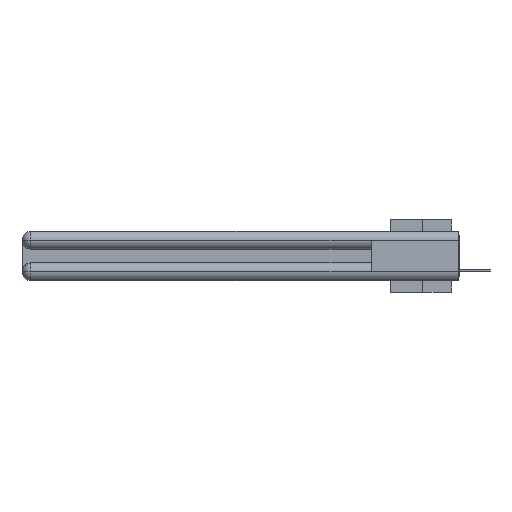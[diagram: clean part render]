
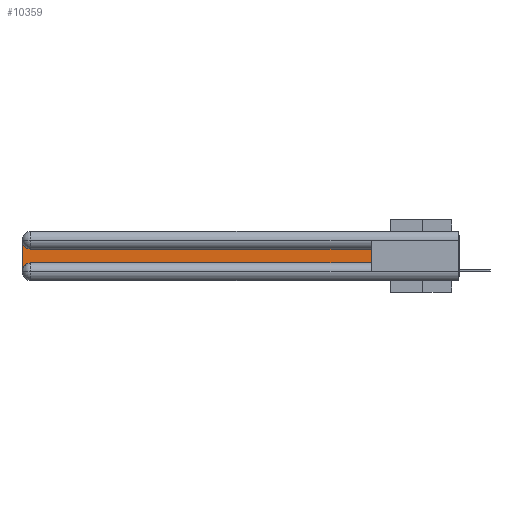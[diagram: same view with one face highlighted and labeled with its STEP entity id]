
A CAD part, left-side view. The second image highlights one B-rep face of the part: STEP entity #10359.
In plain terms, the highlighted planar face has unit normal (-1, 0, 0).
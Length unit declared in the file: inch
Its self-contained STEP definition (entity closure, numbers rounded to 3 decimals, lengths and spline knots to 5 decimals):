
#188 = CARTESIAN_POINT ( 'NONE',  ( 0.075, 3., -0.2175 ) ) ;
#963 = ORIENTED_EDGE ( 'NONE', *, *, #7493, .T. ) ;
#1847 = CARTESIAN_POINT ( 'NONE',  ( 0.075, 2.94, -0.2775 ) ) ;
#2055 = DIRECTION ( 'NONE',  ( 1., 0., 0. ) ) ;
#2234 = LINE ( 'NONE', #188, #9024 ) ;
#4296 = EDGE_CURVE ( 'NONE', #28843, #17159, #2234, .T. ) ;
#6212 = ORIENTED_EDGE ( 'NONE', *, *, #6894, .T. ) ;
#6613 = DIRECTION ( 'NONE',  ( 0., 1., 0. ) ) ;
#6894 = EDGE_CURVE ( 'NONE', #22599, #12963, #25874, .T. ) ;
#7059 = CARTESIAN_POINT ( 'NONE',  ( 0.075, 0.6, -0.2175 ) ) ;
#7493 = EDGE_CURVE ( 'NONE', #19173, #12320, #16929, .T. ) ;
#7584 = LINE ( 'NONE', #29138, #8318 ) ;
#8318 = VECTOR ( 'NONE', #17088, 39.37008 ) ;
#8584 = ORIENTED_EDGE ( 'NONE', *, *, #4296, .T. ) ;
#8745 = DIRECTION ( 'NONE',  ( 0., 0., -1. ) ) ;
#8918 = EDGE_CURVE ( 'NONE', #12320, #28843, #13031, .T. ) ;
#9024 = VECTOR ( 'NONE', #19634, 39.37008 ) ;
#10276 = CARTESIAN_POINT ( 'NONE',  ( 0.075, 0.6, -0.1225 ) ) ;
#10359 = ADVANCED_FACE ( 'NONE', ( #26629 ), #30049, .F. ) ;
#11123 = CARTESIAN_POINT ( 'NONE',  ( 0.075, 3., -0.1225 ) ) ;
#11549 = EDGE_LOOP ( 'NONE', ( #963, #23551, #8584, #31205, #6212, #21942 ) ) ;
#12320 = VERTEX_POINT ( 'NONE', #18294 ) ;
#12775 = VECTOR ( 'NONE', #6613, 39.37008 ) ;
#12963 = VERTEX_POINT ( 'NONE', #20811 ) ;
#13031 = CIRCLE ( 'NONE', #18226, 0.06 ) ;
#13593 = CIRCLE ( 'NONE', #22680, 0.06 ) ;
#16929 = LINE ( 'NONE', #21111, #12775 ) ;
#17088 = DIRECTION ( 'NONE',  ( 0., 0., 1. ) ) ;
#17159 = VERTEX_POINT ( 'NONE', #17723 ) ;
#17723 = CARTESIAN_POINT ( 'NONE',  ( 0.075, 3., -0.2775 ) ) ;
#18226 = AXIS2_PLACEMENT_3D ( 'NONE', #20825, #23264, #8745 ) ;
#18294 = CARTESIAN_POINT ( 'NONE',  ( 0.075, 2.94, -0.1225 ) ) ;
#19173 = VERTEX_POINT ( 'NONE', #10276 ) ;
#19332 = DIRECTION ( 'NONE',  ( 0., -1., 0. ) ) ;
#19634 = DIRECTION ( 'NONE',  ( 0., 0., -1. ) ) ;
#20811 = CARTESIAN_POINT ( 'NONE',  ( 0.075, 0.6, -0.2175 ) ) ;
#20825 = CARTESIAN_POINT ( 'NONE',  ( 0.075, 2.94, -0.0625 ) ) ;
#21111 = CARTESIAN_POINT ( 'NONE',  ( 0.075, 0.6, -0.1225 ) ) ;
#21385 = EDGE_CURVE ( 'NONE', #17159, #22599, #13593, .T. ) ;
#21942 = ORIENTED_EDGE ( 'NONE', *, *, #27292, .T. ) ;
#22599 = VERTEX_POINT ( 'NONE', #26428 ) ;
#22680 = AXIS2_PLACEMENT_3D ( 'NONE', #1847, #2055, #28582 ) ;
#23264 = DIRECTION ( 'NONE',  ( 1., 0., 0. ) ) ;
#23551 = ORIENTED_EDGE ( 'NONE', *, *, #8918, .T. ) ;
#25552 = AXIS2_PLACEMENT_3D ( 'NONE', #11123, #25635, #27744 ) ;
#25635 = DIRECTION ( 'NONE',  ( 1., 0., 0. ) ) ;
#25874 = LINE ( 'NONE', #7059, #29993 ) ;
#26428 = CARTESIAN_POINT ( 'NONE',  ( 0.075, 2.94, -0.2175 ) ) ;
#26629 = FACE_OUTER_BOUND ( 'NONE', #11549, .T. ) ;
#27292 = EDGE_CURVE ( 'NONE', #12963, #19173, #7584, .T. ) ;
#27744 = DIRECTION ( 'NONE',  ( 0., 0., -1. ) ) ;
#28582 = DIRECTION ( 'NONE',  ( 0., 0., -1. ) ) ;
#28843 = VERTEX_POINT ( 'NONE', #30753 ) ;
#29138 = CARTESIAN_POINT ( 'NONE',  ( 0.075, 0.6, -0.2175 ) ) ;
#29993 = VECTOR ( 'NONE', #19332, 39.37008 ) ;
#30049 = PLANE ( 'NONE',  #25552 ) ;
#30753 = CARTESIAN_POINT ( 'NONE',  ( 0.075, 3., -0.0625 ) ) ;
#31205 = ORIENTED_EDGE ( 'NONE', *, *, #21385, .T. ) ;
